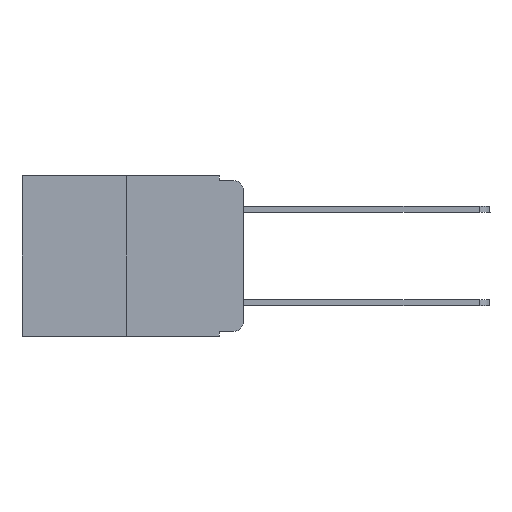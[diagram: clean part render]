
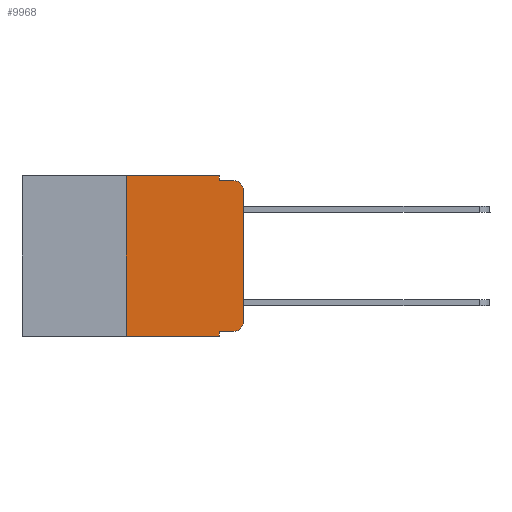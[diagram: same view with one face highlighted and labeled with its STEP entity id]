
A CAD part, left-side view. The second image highlights one B-rep face of the part: STEP entity #9968.
In plain terms, the highlighted planar face has unit normal (-1, 0, 0).
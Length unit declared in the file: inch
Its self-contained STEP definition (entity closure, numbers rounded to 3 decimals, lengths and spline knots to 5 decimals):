
#326 = DIRECTION ( 'NONE',  ( 0., 0., 1. ) ) ;
#623 = CARTESIAN_POINT ( 'NONE',  ( 0., 0.02, -0.03 ) ) ;
#1082 = EDGE_LOOP ( 'NONE', ( #10237, #7861, #17060, #10310, #8908, #16258, #6987, #17941, #14840, #5164 ) ) ;
#1103 = VECTOR ( 'NONE', #7409, 39.37008 ) ;
#1196 = VERTEX_POINT ( 'NONE', #4593 ) ;
#1677 = CARTESIAN_POINT ( 'NONE',  ( 0., 0.25, 0. ) ) ;
#1972 = VERTEX_POINT ( 'NONE', #5578 ) ;
#2396 = CARTESIAN_POINT ( 'NONE',  ( 0., 0.25, -0.343 ) ) ;
#2424 = DIRECTION ( 'NONE',  ( -1., 0., 0. ) ) ;
#2955 = AXIS2_PLACEMENT_3D ( 'NONE', #623, #2424, #15192 ) ;
#2984 = CARTESIAN_POINT ( 'NONE',  ( 0., 0.25, 0. ) ) ;
#3050 = CARTESIAN_POINT ( 'NONE',  ( 0., 0.473, 0. ) ) ;
#3252 = CARTESIAN_POINT ( 'NONE',  ( 0., 0.051, -0.343 ) ) ;
#3322 = EDGE_CURVE ( 'NONE', #10330, #14619, #18320, .T. ) ;
#3502 = VERTEX_POINT ( 'NONE', #3252 ) ;
#3900 = LINE ( 'NONE', #5485, #8976 ) ;
#4593 = CARTESIAN_POINT ( 'NONE',  ( 0., 0.02, -0.01 ) ) ;
#4611 = CARTESIAN_POINT ( 'NONE',  ( 0., 0.051, -0.01 ) ) ;
#4864 = LINE ( 'NONE', #11839, #14976 ) ;
#5080 = LINE ( 'NONE', #6481, #16107 ) ;
#5164 = ORIENTED_EDGE ( 'NONE', *, *, #17732, .T. ) ;
#5324 = CARTESIAN_POINT ( 'NONE',  ( 0., 0.051, 0. ) ) ;
#5424 = CARTESIAN_POINT ( 'NONE',  ( 0., 0., -0.03 ) ) ;
#5485 = CARTESIAN_POINT ( 'NONE',  ( 0., 0.473, -0.343 ) ) ;
#5578 = CARTESIAN_POINT ( 'NONE',  ( 0., 0.02, -0.333 ) ) ;
#6481 = CARTESIAN_POINT ( 'NONE',  ( 0., 0.051, 0. ) ) ;
#6987 = ORIENTED_EDGE ( 'NONE', *, *, #15813, .T. ) ;
#7035 = AXIS2_PLACEMENT_3D ( 'NONE', #3050, #8787, #14508 ) ;
#7081 = VECTOR ( 'NONE', #17157, 39.37008 ) ;
#7409 = DIRECTION ( 'NONE',  ( 0., 0., 1. ) ) ;
#7428 = DIRECTION ( 'NONE',  ( -1., 0., 0. ) ) ;
#7585 = EDGE_CURVE ( 'NONE', #14619, #1196, #9321, .T. ) ;
#7670 = VERTEX_POINT ( 'NONE', #9226 ) ;
#7810 = DIRECTION ( 'NONE',  ( 0., -1., 0. ) ) ;
#7851 = VECTOR ( 'NONE', #7810, 39.37008 ) ;
#7861 = ORIENTED_EDGE ( 'NONE', *, *, #13519, .T. ) ;
#8787 = DIRECTION ( 'NONE',  ( 1., 0., 0. ) ) ;
#8820 = EDGE_CURVE ( 'NONE', #12472, #3502, #5080, .T. ) ;
#8908 = ORIENTED_EDGE ( 'NONE', *, *, #16634, .F. ) ;
#8976 = VECTOR ( 'NONE', #11133, 39.37008 ) ;
#8981 = DIRECTION ( 'NONE',  ( 0., -1., 0. ) ) ;
#9152 = CARTESIAN_POINT ( 'NONE',  ( 0., 0.051, -0.333 ) ) ;
#9226 = CARTESIAN_POINT ( 'NONE',  ( 0., 0., -0.313 ) ) ;
#9321 = LINE ( 'NONE', #17860, #7851 ) ;
#9412 = VERTEX_POINT ( 'NONE', #5424 ) ;
#9513 = VERTEX_POINT ( 'NONE', #2984 ) ;
#9724 = VERTEX_POINT ( 'NONE', #2396 ) ;
#9968 = ADVANCED_FACE ( 'NONE', ( #10188 ), #15907, .F. ) ;
#10188 = FACE_OUTER_BOUND ( 'NONE', #1082, .T. ) ;
#10237 = ORIENTED_EDGE ( 'NONE', *, *, #12651, .T. ) ;
#10310 = ORIENTED_EDGE ( 'NONE', *, *, #3322, .F. ) ;
#10330 = VERTEX_POINT ( 'NONE', #14396 ) ;
#10601 = DIRECTION ( 'NONE',  ( 0., -1., 0. ) ) ;
#11040 = VECTOR ( 'NONE', #8981, 39.37008 ) ;
#11133 = DIRECTION ( 'NONE',  ( 0., -1., 0. ) ) ;
#11839 = CARTESIAN_POINT ( 'NONE',  ( 0., 0.473, 0. ) ) ;
#12265 = EDGE_CURVE ( 'NONE', #9724, #9513, #16229, .T. ) ;
#12472 = VERTEX_POINT ( 'NONE', #15849 ) ;
#12651 = EDGE_CURVE ( 'NONE', #7670, #9412, #13215, .T. ) ;
#12996 = EDGE_CURVE ( 'NONE', #12472, #1972, #16556, .T. ) ;
#13215 = LINE ( 'NONE', #17531, #14024 ) ;
#13337 = DIRECTION ( 'NONE',  ( 0., 0., -1. ) ) ;
#13519 = EDGE_CURVE ( 'NONE', #9412, #1196, #18571, .T. ) ;
#14024 = VECTOR ( 'NONE', #326, 39.37008 ) ;
#14396 = CARTESIAN_POINT ( 'NONE',  ( 0., 0.051, 0. ) ) ;
#14508 = DIRECTION ( 'NONE',  ( 0., 0., -1. ) ) ;
#14619 = VERTEX_POINT ( 'NONE', #4611 ) ;
#14840 = ORIENTED_EDGE ( 'NONE', *, *, #12996, .T. ) ;
#14976 = VECTOR ( 'NONE', #10601, 39.37008 ) ;
#15001 = CIRCLE ( 'NONE', #18350, 0.02 ) ;
#15113 = DIRECTION ( 'NONE',  ( 0., 0., -1. ) ) ;
#15192 = DIRECTION ( 'NONE',  ( 0., 0., -1. ) ) ;
#15813 = EDGE_CURVE ( 'NONE', #9724, #3502, #3900, .T. ) ;
#15849 = CARTESIAN_POINT ( 'NONE',  ( 0., 0.051, -0.333 ) ) ;
#15907 = PLANE ( 'NONE',  #7035 ) ;
#16062 = CARTESIAN_POINT ( 'NONE',  ( 0., 0.02, -0.313 ) ) ;
#16107 = VECTOR ( 'NONE', #15113, 39.37008 ) ;
#16229 = LINE ( 'NONE', #1677, #1103 ) ;
#16258 = ORIENTED_EDGE ( 'NONE', *, *, #12265, .F. ) ;
#16556 = LINE ( 'NONE', #9152, #11040 ) ;
#16634 = EDGE_CURVE ( 'NONE', #9513, #10330, #4864, .T. ) ;
#17060 = ORIENTED_EDGE ( 'NONE', *, *, #7585, .F. ) ;
#17157 = DIRECTION ( 'NONE',  ( 0., 0., -1. ) ) ;
#17531 = CARTESIAN_POINT ( 'NONE',  ( 0., 0., 0. ) ) ;
#17732 = EDGE_CURVE ( 'NONE', #1972, #7670, #15001, .T. ) ;
#17860 = CARTESIAN_POINT ( 'NONE',  ( 0., 0.051, -0.01 ) ) ;
#17941 = ORIENTED_EDGE ( 'NONE', *, *, #8820, .F. ) ;
#18320 = LINE ( 'NONE', #5324, #7081 ) ;
#18350 = AXIS2_PLACEMENT_3D ( 'NONE', #16062, #7428, #13337 ) ;
#18571 = CIRCLE ( 'NONE', #2955, 0.02 ) ;
